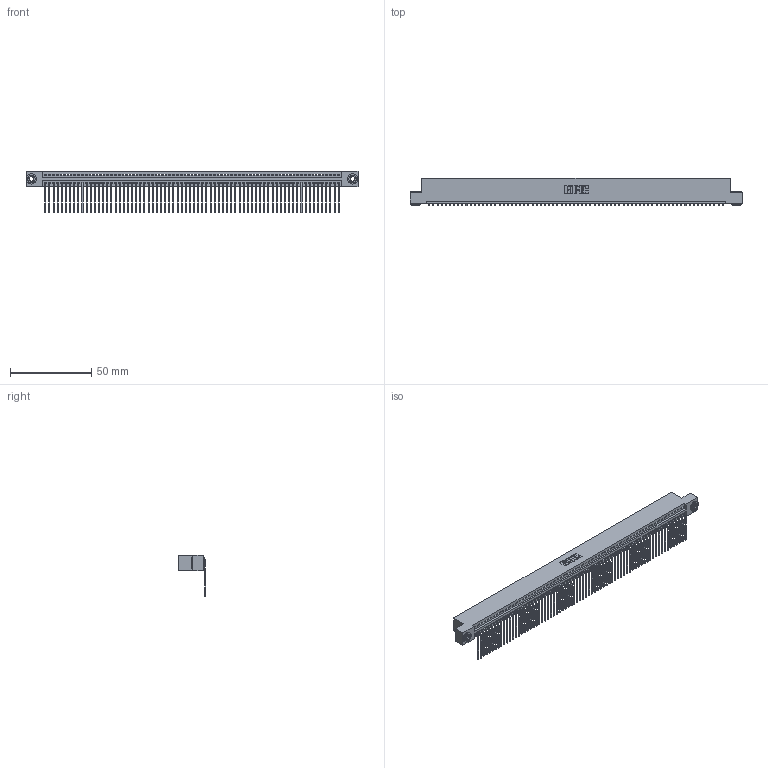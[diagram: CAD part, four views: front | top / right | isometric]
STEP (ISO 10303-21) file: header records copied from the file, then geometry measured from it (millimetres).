
FILE_DESCRIPTION (( 'STEP AP203' ), '1' );
FILE_NAME ('345-072-559-103.STEP', '2019-10-15T12:12:25', ( '' ), ( '' ), 'SwSTEP 2.0', 'SolidWorks 2016', '' );
FILE_SCHEMA (( 'CONFIG_CONTROL_DESIGN' ));
Length unit declared in the file: inch
Products named in the file (4): 345-250-002_345-250-002-102; 345-292-001_558 559 Tail - 1; 345 Part_Flush Mounting Lugs - 0.156 Dia-TH; 345-072-559-103
Assembly tree (75 placements, depth 2):
  345-072-559-103
    345 Part_Flush Mounting Lugs - 0.156 Dia-TH
    345-292-001_558 559 Tail - 1  x72
    345-250-002_345-250-002-102  x2
Bounding box: 204.09 x 16.75 x 25.53 mm (x, y, z)
Volume: 19889.6 mm3; surface area: 28463.3 mm2
Topology: 75 solids, 75 shells, 4484 faces, 13521 edges, 8914 vertices
Faces by surface type: plane 3114, cylinder 1362, cone 8
Entity records: 50884 total; most frequent: CARTESIAN_POINT 8791, ORIENTED_EDGE 8790, DIRECTION 7665, EDGE_CURVE 4395, LINE 3951, VECTOR 3951, VERTEX_POINT 2926, AXIS2_PLACEMENT_3D 1857
